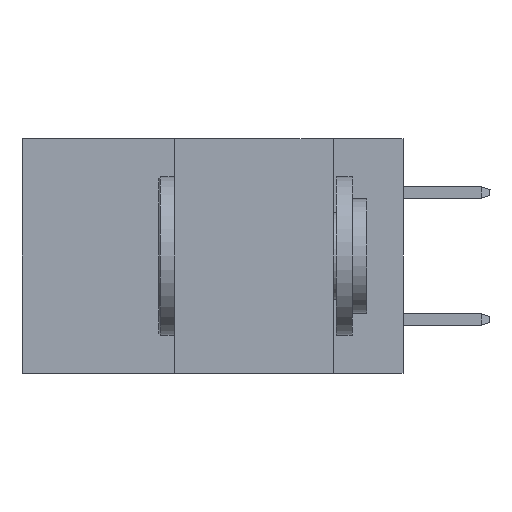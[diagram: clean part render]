
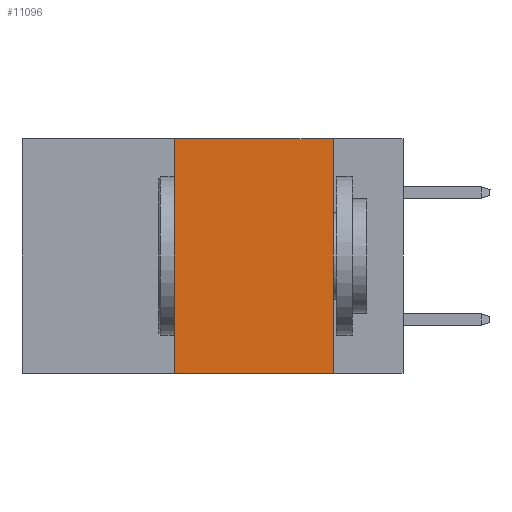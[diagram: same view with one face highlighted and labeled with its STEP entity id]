
A CAD part, left-side view. The second image highlights one B-rep face of the part: STEP entity #11096.
In plain terms, the highlighted planar face has unit normal (-1, 0, 0).
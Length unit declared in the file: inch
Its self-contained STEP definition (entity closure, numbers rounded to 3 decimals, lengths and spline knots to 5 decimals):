
#457 = CARTESIAN_POINT ( 'NONE',  ( 0., 0.11, 0. ) ) ;
#498 = LINE ( 'NONE', #1718, #1125 ) ;
#1081 = VERTEX_POINT ( 'NONE', #16432 ) ;
#1125 = VECTOR ( 'NONE', #6660, 39.37008 ) ;
#1543 = VECTOR ( 'NONE', #6257, 39.37008 ) ;
#1718 = CARTESIAN_POINT ( 'NONE',  ( 0., 0.6, -0.37 ) ) ;
#1982 = AXIS2_PLACEMENT_3D ( 'NONE', #11853, #12067, #10325 ) ;
#2260 = EDGE_LOOP ( 'NONE', ( #5994, #11885, #4629, #11760 ) ) ;
#3631 = CARTESIAN_POINT ( 'NONE',  ( 0., 0.11, 0. ) ) ;
#4572 = LINE ( 'NONE', #11140, #1543 ) ;
#4629 = ORIENTED_EDGE ( 'NONE', *, *, #20827, .F. ) ;
#5460 = LINE ( 'NONE', #3631, #13635 ) ;
#5994 = ORIENTED_EDGE ( 'NONE', *, *, #19985, .F. ) ;
#6257 = DIRECTION ( 'NONE',  ( 0., 0., 1. ) ) ;
#6336 = DIRECTION ( 'NONE',  ( 0., -1., 0. ) ) ;
#6438 = CARTESIAN_POINT ( 'NONE',  ( 0., 0.6, 0. ) ) ;
#6660 = DIRECTION ( 'NONE',  ( 0., -1., 0. ) ) ;
#8886 = EDGE_CURVE ( 'NONE', #1081, #9425, #19631, .T. ) ;
#9114 = VERTEX_POINT ( 'NONE', #20723 ) ;
#9425 = VERTEX_POINT ( 'NONE', #457 ) ;
#10015 = VERTEX_POINT ( 'NONE', #12873 ) ;
#10325 = DIRECTION ( 'NONE',  ( 0., 0., -1. ) ) ;
#11096 = ADVANCED_FACE ( 'NONE', ( #17073 ), #20365, .F. ) ;
#11140 = CARTESIAN_POINT ( 'NONE',  ( 0., 0.36, 0. ) ) ;
#11760 = ORIENTED_EDGE ( 'NONE', *, *, #16104, .T. ) ;
#11853 = CARTESIAN_POINT ( 'NONE',  ( 0., 0.6, 0. ) ) ;
#11885 = ORIENTED_EDGE ( 'NONE', *, *, #8886, .F. ) ;
#12067 = DIRECTION ( 'NONE',  ( 1., 0., 0. ) ) ;
#12739 = VECTOR ( 'NONE', #6336, 39.37008 ) ;
#12873 = CARTESIAN_POINT ( 'NONE',  ( 0., 0.11, -0.37 ) ) ;
#13635 = VECTOR ( 'NONE', #16847, 39.37008 ) ;
#16104 = EDGE_CURVE ( 'NONE', #9114, #10015, #498, .T. ) ;
#16432 = CARTESIAN_POINT ( 'NONE',  ( 0., 0.36, 0. ) ) ;
#16847 = DIRECTION ( 'NONE',  ( 0., 0., -1. ) ) ;
#17073 = FACE_OUTER_BOUND ( 'NONE', #2260, .T. ) ;
#19631 = LINE ( 'NONE', #6438, #12739 ) ;
#19985 = EDGE_CURVE ( 'NONE', #9425, #10015, #5460, .T. ) ;
#20365 = PLANE ( 'NONE',  #1982 ) ;
#20723 = CARTESIAN_POINT ( 'NONE',  ( 0., 0.36, -0.37 ) ) ;
#20827 = EDGE_CURVE ( 'NONE', #9114, #1081, #4572, .T. ) ;
